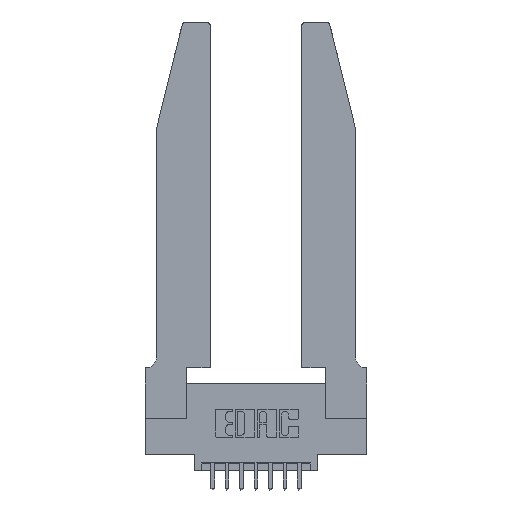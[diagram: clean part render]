
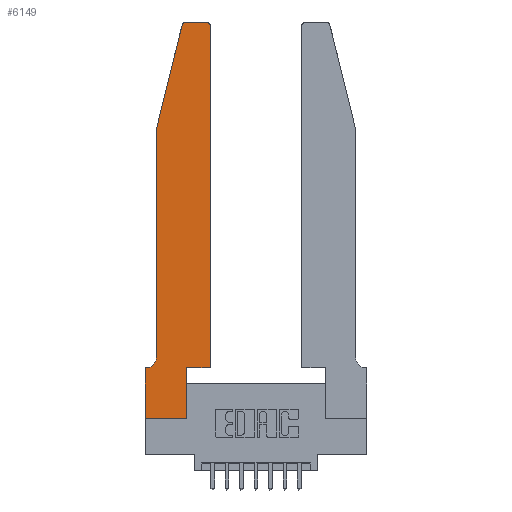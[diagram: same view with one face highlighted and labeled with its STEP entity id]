
A CAD part, top view. The second image highlights one B-rep face of the part: STEP entity #6149.
In plain terms, the highlighted planar face has unit normal (0, 0, 1).
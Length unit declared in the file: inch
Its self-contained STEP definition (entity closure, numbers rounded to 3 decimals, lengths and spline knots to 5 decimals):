
#139 = VECTOR ( 'NONE', #12972, 39.37008 ) ;
#171 = ORIENTED_EDGE ( 'NONE', *, *, #4028, .T. ) ;
#536 = ORIENTED_EDGE ( 'NONE', *, *, #14486, .T. ) ;
#918 = EDGE_CURVE ( 'NONE', #6253, #1454, #5172, .T. ) ;
#931 = CARTESIAN_POINT ( 'NONE',  ( 0., 0., 0.37 ) ) ;
#984 = VECTOR ( 'NONE', #9409, 39.37008 ) ;
#1454 = VERTEX_POINT ( 'NONE', #10300 ) ;
#1484 = AXIS2_PLACEMENT_3D ( 'NONE', #3532, #6669, #3442 ) ;
#1487 = CARTESIAN_POINT ( 'NONE',  ( 0.4505, 0.35, 0.37 ) ) ;
#1634 = LINE ( 'NONE', #14121, #12942 ) ;
#1640 = EDGE_CURVE ( 'NONE', #1454, #8416, #2752, .T. ) ;
#1957 = AXIS2_PLACEMENT_3D ( 'NONE', #13261, #12123, #14235 ) ;
#2133 = CARTESIAN_POINT ( 'NONE',  ( 0., 0.35, 0.37 ) ) ;
#2173 = LINE ( 'NONE', #8203, #6699 ) ;
#2253 = ORIENTED_EDGE ( 'NONE', *, *, #3728, .T. ) ;
#2448 = CARTESIAN_POINT ( 'NONE',  ( 0.284, 2.75, 0.37 ) ) ;
#2708 = DIRECTION ( 'NONE',  ( 0., 0., 1. ) ) ;
#2734 = DIRECTION ( 'NONE',  ( 1., 0., 0. ) ) ;
#2752 = LINE ( 'NONE', #5828, #139 ) ;
#2894 = EDGE_CURVE ( 'NONE', #11698, #4435, #1634, .T. ) ;
#3156 = CIRCLE ( 'NONE', #1957, 0.07 ) ;
#3378 = VECTOR ( 'NONE', #14737, 39.37008 ) ;
#3431 = CARTESIAN_POINT ( 'NONE',  ( 0.4505, 0.35, 0.37 ) ) ;
#3442 = DIRECTION ( 'NONE',  ( 1., 0., 0. ) ) ;
#3463 = DIRECTION ( 'NONE',  ( 0., 0., 1. ) ) ;
#3464 = LINE ( 'NONE', #11071, #11340 ) ;
#3532 = CARTESIAN_POINT ( 'NONE',  ( 0.4205, 2.72, 0.37 ) ) ;
#3636 = VECTOR ( 'NONE', #5814, 39.37008 ) ;
#3728 = EDGE_CURVE ( 'NONE', #9972, #8424, #6110, .T. ) ;
#4028 = EDGE_CURVE ( 'NONE', #8416, #7495, #5375, .T. ) ;
#4435 = VERTEX_POINT ( 'NONE', #11919 ) ;
#4939 = DIRECTION ( 'NONE',  ( 1., 0., 0. ) ) ;
#5024 = DIRECTION ( 'NONE',  ( -1., 0., 0. ) ) ;
#5172 = CIRCLE ( 'NONE', #1484, 0.03 ) ;
#5375 = CIRCLE ( 'NONE', #8703, 0.03 ) ;
#5470 = CARTESIAN_POINT ( 'NONE',  ( 0.0755, 0.42, 0.37 ) ) ;
#5516 = VERTEX_POINT ( 'NONE', #3431 ) ;
#5657 = ORIENTED_EDGE ( 'NONE', *, *, #14568, .T. ) ;
#5814 = DIRECTION ( 'NONE',  ( 0., -1., 0. ) ) ;
#5828 = CARTESIAN_POINT ( 'NONE',  ( 0.2605, 2.75, 0.37 ) ) ;
#5851 = PLANE ( 'NONE',  #8735 ) ;
#6055 = CARTESIAN_POINT ( 'NONE',  ( 0.4505, 2.72, 0.37 ) ) ;
#6110 = LINE ( 'NONE', #931, #3378 ) ;
#6149 = ADVANCED_FACE ( 'NONE', ( #8479 ), #5851, .T. ) ;
#6253 = VERTEX_POINT ( 'NONE', #6055 ) ;
#6302 = ORIENTED_EDGE ( 'NONE', *, *, #10071, .T. ) ;
#6519 = VECTOR ( 'NONE', #5024, 39.37008 ) ;
#6669 = DIRECTION ( 'NONE',  ( 0., 0., 1. ) ) ;
#6699 = VECTOR ( 'NONE', #10543, 39.37008 ) ;
#6935 = ORIENTED_EDGE ( 'NONE', *, *, #9494, .T. ) ;
#6994 = DIRECTION ( 'NONE',  ( 1., 0., 0. ) ) ;
#7495 = VERTEX_POINT ( 'NONE', #14835 ) ;
#7498 = ORIENTED_EDGE ( 'NONE', *, *, #12388, .T. ) ;
#8190 = LINE ( 'NONE', #9468, #3636 ) ;
#8203 = CARTESIAN_POINT ( 'NONE',  ( 0., 0., 0.37 ) ) ;
#8416 = VERTEX_POINT ( 'NONE', #2448 ) ;
#8424 = VERTEX_POINT ( 'NONE', #12947 ) ;
#8479 = FACE_OUTER_BOUND ( 'NONE', #8757, .T. ) ;
#8703 = AXIS2_PLACEMENT_3D ( 'NONE', #11965, #2708, #4939 ) ;
#8735 = AXIS2_PLACEMENT_3D ( 'NONE', #11644, #3463, #6994 ) ;
#8757 = EDGE_LOOP ( 'NONE', ( #10751, #171, #5657, #6302, #14332, #7498, #2253, #9523, #13394, #536, #6935, #12111 ) ) ;
#8897 = LINE ( 'NONE', #14387, #6519 ) ;
#9409 = DIRECTION ( 'NONE',  ( 0., 1., 0. ) ) ;
#9447 = DIRECTION ( 'NONE',  ( 0., 1., 0. ) ) ;
#9468 = CARTESIAN_POINT ( 'NONE',  ( 0.0755, 2., 0.37 ) ) ;
#9494 = EDGE_CURVE ( 'NONE', #5516, #6253, #14884, .T. ) ;
#9523 = ORIENTED_EDGE ( 'NONE', *, *, #12822, .T. ) ;
#9546 = EDGE_CURVE ( 'NONE', #14233, #11606, #3156, .T. ) ;
#9972 = VERTEX_POINT ( 'NONE', #2133 ) ;
#10071 = EDGE_CURVE ( 'NONE', #11914, #14233, #8190, .T. ) ;
#10300 = CARTESIAN_POINT ( 'NONE',  ( 0.4205, 2.75, 0.37 ) ) ;
#10368 = CARTESIAN_POINT ( 'NONE',  ( 0.0755, 2., 0.37 ) ) ;
#10543 = DIRECTION ( 'NONE',  ( 1., 0., 0. ) ) ;
#10751 = ORIENTED_EDGE ( 'NONE', *, *, #1640, .T. ) ;
#10981 = VECTOR ( 'NONE', #11848, 39.37008 ) ;
#11071 = CARTESIAN_POINT ( 'NONE',  ( 0.4505, 0.35, 0.37 ) ) ;
#11152 = CARTESIAN_POINT ( 'NONE',  ( 0.0055, 0.35, 0.37 ) ) ;
#11340 = VECTOR ( 'NONE', #2734, 39.37008 ) ;
#11606 = VERTEX_POINT ( 'NONE', #11152 ) ;
#11644 = CARTESIAN_POINT ( 'NONE',  ( 0., 0.35, 0.37 ) ) ;
#11698 = VERTEX_POINT ( 'NONE', #12163 ) ;
#11848 = DIRECTION ( 'NONE',  ( -0.239, -0.971, 0. ) ) ;
#11895 = LINE ( 'NONE', #10368, #10981 ) ;
#11914 = VERTEX_POINT ( 'NONE', #13029 ) ;
#11919 = CARTESIAN_POINT ( 'NONE',  ( 0.2865, 0.35, 0.37 ) ) ;
#11965 = CARTESIAN_POINT ( 'NONE',  ( 0.284, 2.72, 0.37 ) ) ;
#12111 = ORIENTED_EDGE ( 'NONE', *, *, #918, .T. ) ;
#12123 = DIRECTION ( 'NONE',  ( 0., 0., -1. ) ) ;
#12163 = CARTESIAN_POINT ( 'NONE',  ( 0.2865, 0., 0.37 ) ) ;
#12388 = EDGE_CURVE ( 'NONE', #11606, #9972, #8897, .T. ) ;
#12822 = EDGE_CURVE ( 'NONE', #8424, #11698, #2173, .T. ) ;
#12942 = VECTOR ( 'NONE', #9447, 39.37008 ) ;
#12947 = CARTESIAN_POINT ( 'NONE',  ( 0., 0., 0.37 ) ) ;
#12972 = DIRECTION ( 'NONE',  ( -1., 0., 0. ) ) ;
#13029 = CARTESIAN_POINT ( 'NONE',  ( 0.0755, 2., 0.37 ) ) ;
#13261 = CARTESIAN_POINT ( 'NONE',  ( 0.0055, 0.42, 0.37 ) ) ;
#13394 = ORIENTED_EDGE ( 'NONE', *, *, #2894, .T. ) ;
#14121 = CARTESIAN_POINT ( 'NONE',  ( 0.2865, 0.35, 0.37 ) ) ;
#14233 = VERTEX_POINT ( 'NONE', #5470 ) ;
#14235 = DIRECTION ( 'NONE',  ( -1., 0., 0. ) ) ;
#14332 = ORIENTED_EDGE ( 'NONE', *, *, #9546, .T. ) ;
#14387 = CARTESIAN_POINT ( 'NONE',  ( 0.0755, 0.35, 0.37 ) ) ;
#14486 = EDGE_CURVE ( 'NONE', #4435, #5516, #3464, .T. ) ;
#14568 = EDGE_CURVE ( 'NONE', #7495, #11914, #11895, .T. ) ;
#14737 = DIRECTION ( 'NONE',  ( 0., -1., 0. ) ) ;
#14835 = CARTESIAN_POINT ( 'NONE',  ( 0.25487, 2.72718, 0.37 ) ) ;
#14884 = LINE ( 'NONE', #1487, #984 ) ;
